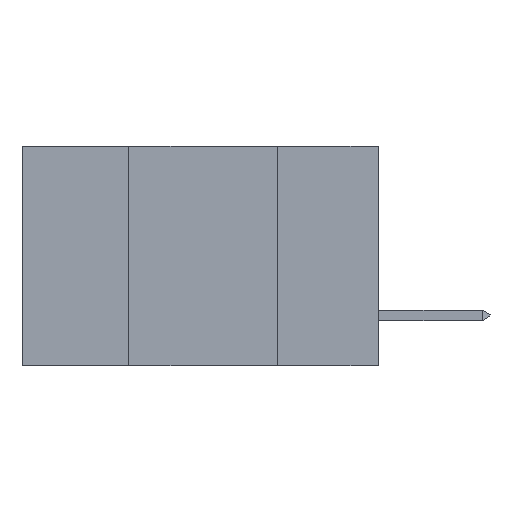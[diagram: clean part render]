
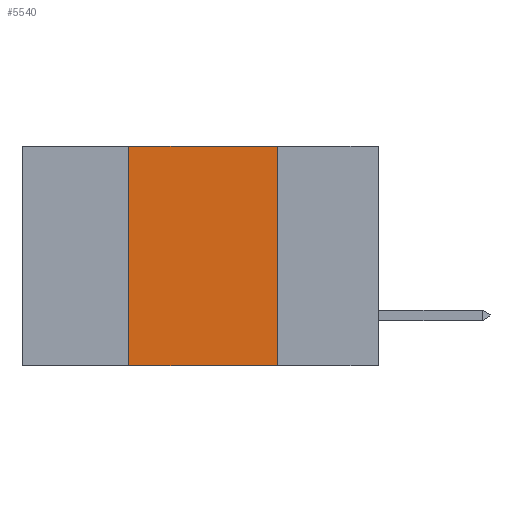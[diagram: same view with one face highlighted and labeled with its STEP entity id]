
A CAD part, left-side view. The second image highlights one B-rep face of the part: STEP entity #5540.
In plain terms, the highlighted planar face has unit normal (-1, 0, 0).
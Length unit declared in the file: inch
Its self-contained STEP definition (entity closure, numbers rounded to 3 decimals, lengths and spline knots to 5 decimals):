
#1369 = CARTESIAN_POINT ( 'NONE',  ( 0., 0.42, 0. ) ) ;
#1537 = DIRECTION ( 'NONE',  ( 0., -1., 0. ) ) ;
#1892 = VECTOR ( 'NONE', #10897, 39.37008 ) ;
#2961 = CARTESIAN_POINT ( 'NONE',  ( 0., 0.17, 0. ) ) ;
#3088 = CARTESIAN_POINT ( 'NONE',  ( 0., 0.6, 0. ) ) ;
#3284 = LINE ( 'NONE', #19294, #4663 ) ;
#4663 = VECTOR ( 'NONE', #1537, 39.37008 ) ;
#4869 = AXIS2_PLACEMENT_3D ( 'NONE', #3088, #22478, #15475 ) ;
#4983 = DIRECTION ( 'NONE',  ( 0., 0., 1. ) ) ;
#5540 = ADVANCED_FACE ( 'NONE', ( #21548 ), #6586, .F. ) ;
#5596 = DIRECTION ( 'NONE',  ( 0., 0., -1. ) ) ;
#5631 = ORIENTED_EDGE ( 'NONE', *, *, #15476, .T. ) ;
#5933 = VERTEX_POINT ( 'NONE', #1369 ) ;
#6586 = PLANE ( 'NONE',  #4869 ) ;
#6864 = VECTOR ( 'NONE', #4983, 39.37008 ) ;
#7813 = VERTEX_POINT ( 'NONE', #20542 ) ;
#8438 = VECTOR ( 'NONE', #5596, 39.37008 ) ;
#9317 = CARTESIAN_POINT ( 'NONE',  ( 0., 0.17, 0. ) ) ;
#9850 = ORIENTED_EDGE ( 'NONE', *, *, #17470, .F. ) ;
#10897 = DIRECTION ( 'NONE',  ( 0., -1., 0. ) ) ;
#11442 = CARTESIAN_POINT ( 'NONE',  ( 0., 0.42, -0.37 ) ) ;
#11782 = EDGE_LOOP ( 'NONE', ( #9850, #21031, #11893, #5631 ) ) ;
#11893 = ORIENTED_EDGE ( 'NONE', *, *, #15915, .F. ) ;
#13138 = LINE ( 'NONE', #9317, #8438 ) ;
#14826 = VERTEX_POINT ( 'NONE', #11442 ) ;
#15475 = DIRECTION ( 'NONE',  ( 0., 0., -1. ) ) ;
#15476 = EDGE_CURVE ( 'NONE', #14826, #7813, #3284, .T. ) ;
#15915 = EDGE_CURVE ( 'NONE', #14826, #5933, #19566, .T. ) ;
#17470 = EDGE_CURVE ( 'NONE', #20295, #7813, #13138, .T. ) ;
#17512 = CARTESIAN_POINT ( 'NONE',  ( 0., 0.42, 0. ) ) ;
#19294 = CARTESIAN_POINT ( 'NONE',  ( 0., 0.6, -0.37 ) ) ;
#19566 = LINE ( 'NONE', #17512, #6864 ) ;
#20295 = VERTEX_POINT ( 'NONE', #2961 ) ;
#20542 = CARTESIAN_POINT ( 'NONE',  ( 0., 0.17, -0.37 ) ) ;
#21031 = ORIENTED_EDGE ( 'NONE', *, *, #21847, .F. ) ;
#21235 = LINE ( 'NONE', #21458, #1892 ) ;
#21458 = CARTESIAN_POINT ( 'NONE',  ( 0., 0.6, 0. ) ) ;
#21548 = FACE_OUTER_BOUND ( 'NONE', #11782, .T. ) ;
#21847 = EDGE_CURVE ( 'NONE', #5933, #20295, #21235, .T. ) ;
#22478 = DIRECTION ( 'NONE',  ( 1., 0., 0. ) ) ;
